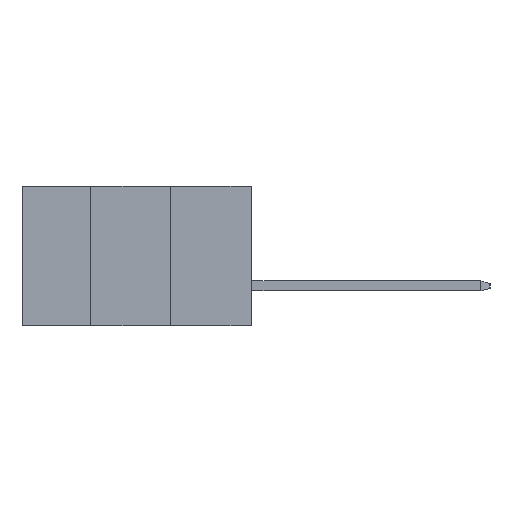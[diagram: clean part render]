
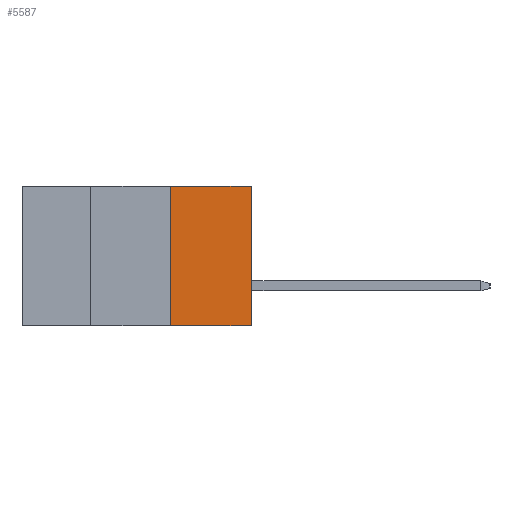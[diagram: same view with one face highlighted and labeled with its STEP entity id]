
A CAD part, left-side view. The second image highlights one B-rep face of the part: STEP entity #5587.
In plain terms, the highlighted planar face has unit normal (-1, 0, 0).
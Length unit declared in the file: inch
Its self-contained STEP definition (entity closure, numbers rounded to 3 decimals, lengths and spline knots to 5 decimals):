
#94 = CARTESIAN_POINT ( 'NONE',  ( 0.4265, 0., 0. ) ) ;
#603 = CARTESIAN_POINT ( 'NONE',  ( 0.4265, 0.254, 0. ) ) ;
#847 = PLANE ( 'NONE',  #5909 ) ;
#1273 = EDGE_CURVE ( 'NONE', #4872, #9298, #7186, .T. ) ;
#2046 = CARTESIAN_POINT ( 'NONE',  ( 0.4265, 0.254, -0.437 ) ) ;
#2317 = VECTOR ( 'NONE', #4783, 39.37008 ) ;
#2955 = DIRECTION ( 'NONE',  ( 0., -1., 0. ) ) ;
#3376 = FACE_OUTER_BOUND ( 'NONE', #7234, .T. ) ;
#3416 = CARTESIAN_POINT ( 'NONE',  ( 0.4265, 0., -0.437 ) ) ;
#3485 = LINE ( 'NONE', #9681, #9217 ) ;
#3536 = EDGE_CURVE ( 'NONE', #4872, #9117, #3485, .T. ) ;
#3923 = EDGE_CURVE ( 'NONE', #9298, #8771, #11420, .T. ) ;
#4398 = CARTESIAN_POINT ( 'NONE',  ( 0.4265, 0.254, -0.437 ) ) ;
#4606 = ORIENTED_EDGE ( 'NONE', *, *, #3923, .T. ) ;
#4723 = CARTESIAN_POINT ( 'NONE',  ( 0.4265, 0.254, -0.437 ) ) ;
#4783 = DIRECTION ( 'NONE',  ( 0., -1., 0. ) ) ;
#4872 = VERTEX_POINT ( 'NONE', #2046 ) ;
#5213 = ORIENTED_EDGE ( 'NONE', *, *, #3536, .F. ) ;
#5587 = ADVANCED_FACE ( 'NONE', ( #3376 ), #847, .F. ) ;
#5909 = AXIS2_PLACEMENT_3D ( 'NONE', #4398, #9367, #7024 ) ;
#6188 = VECTOR ( 'NONE', #2955, 39.37008 ) ;
#7024 = DIRECTION ( 'NONE',  ( 0., 0., -1. ) ) ;
#7186 = LINE ( 'NONE', #4723, #6188 ) ;
#7234 = EDGE_LOOP ( 'NONE', ( #4606, #8609, #5213, #9330 ) ) ;
#7465 = LINE ( 'NONE', #603, #2317 ) ;
#8609 = ORIENTED_EDGE ( 'NONE', *, *, #11356, .F. ) ;
#8682 = VECTOR ( 'NONE', #10718, 39.37008 ) ;
#8771 = VERTEX_POINT ( 'NONE', #94 ) ;
#9117 = VERTEX_POINT ( 'NONE', #9884 ) ;
#9217 = VECTOR ( 'NONE', #9800, 39.37008 ) ;
#9298 = VERTEX_POINT ( 'NONE', #10116 ) ;
#9330 = ORIENTED_EDGE ( 'NONE', *, *, #1273, .T. ) ;
#9367 = DIRECTION ( 'NONE',  ( 1., 0., 0. ) ) ;
#9681 = CARTESIAN_POINT ( 'NONE',  ( 0.4265, 0.254, -0.437 ) ) ;
#9800 = DIRECTION ( 'NONE',  ( 0., 0., 1. ) ) ;
#9884 = CARTESIAN_POINT ( 'NONE',  ( 0.4265, 0.254, 0. ) ) ;
#10116 = CARTESIAN_POINT ( 'NONE',  ( 0.4265, 0., -0.437 ) ) ;
#10718 = DIRECTION ( 'NONE',  ( 0., 0., 1. ) ) ;
#11356 = EDGE_CURVE ( 'NONE', #9117, #8771, #7465, .T. ) ;
#11420 = LINE ( 'NONE', #3416, #8682 ) ;
